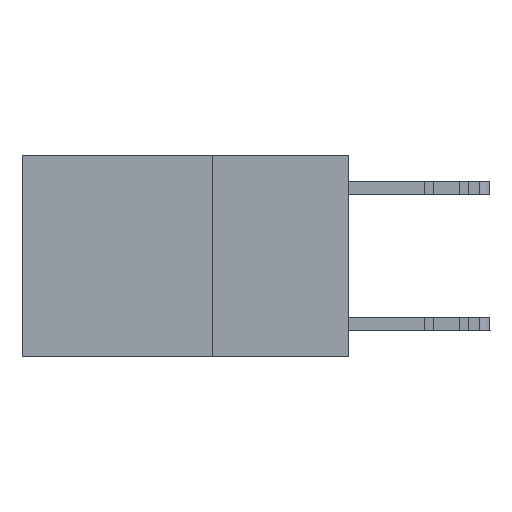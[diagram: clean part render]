
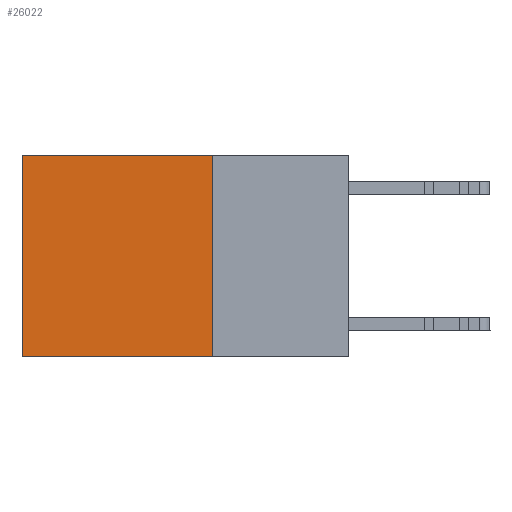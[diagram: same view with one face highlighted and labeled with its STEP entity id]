
A CAD part, left-side view. The second image highlights one B-rep face of the part: STEP entity #26022.
In plain terms, the highlighted planar face has unit normal (-1, 0, 0).
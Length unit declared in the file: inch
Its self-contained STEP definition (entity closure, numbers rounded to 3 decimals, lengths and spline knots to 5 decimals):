
#2023 = CARTESIAN_POINT ( 'NONE',  ( 0.2625, 0.6, 0. ) ) ;
#2108 = PLANE ( 'NONE',  #25555 ) ;
#2206 = ORIENTED_EDGE ( 'NONE', *, *, #14690, .T. ) ;
#4691 = DIRECTION ( 'NONE',  ( 0., 0., -1. ) ) ;
#6877 = ORIENTED_EDGE ( 'NONE', *, *, #31865, .T. ) ;
#6897 = CARTESIAN_POINT ( 'NONE',  ( 0.2625, 0.25, 0. ) ) ;
#7633 = VERTEX_POINT ( 'NONE', #20233 ) ;
#9409 = EDGE_CURVE ( 'NONE', #23916, #25030, #17758, .T. ) ;
#9437 = VERTEX_POINT ( 'NONE', #6897 ) ;
#10968 = LINE ( 'NONE', #23089, #26407 ) ;
#11083 = EDGE_LOOP ( 'NONE', ( #6877, #31672, #31419, #2206 ) ) ;
#12290 = FACE_OUTER_BOUND ( 'NONE', #11083, .T. ) ;
#14148 = DIRECTION ( 'NONE',  ( 0., 0., -1. ) ) ;
#14690 = EDGE_CURVE ( 'NONE', #9437, #7633, #10968, .T. ) ;
#15938 = CARTESIAN_POINT ( 'NONE',  ( 0.2625, 0.25, -0.37 ) ) ;
#16152 = DIRECTION ( 'NONE',  ( 0., 1., 0. ) ) ;
#16973 = VECTOR ( 'NONE', #14148, 39.37008 ) ;
#16997 = CARTESIAN_POINT ( 'NONE',  ( 0.2625, 0.25, 0. ) ) ;
#17758 = LINE ( 'NONE', #23254, #30522 ) ;
#18990 = LINE ( 'NONE', #2023, #16973 ) ;
#20233 = CARTESIAN_POINT ( 'NONE',  ( 0.2625, 0.6, 0. ) ) ;
#22147 = CARTESIAN_POINT ( 'NONE',  ( 0.2625, 0.25, 0. ) ) ;
#23089 = CARTESIAN_POINT ( 'NONE',  ( 0.2625, 0.25, 0. ) ) ;
#23254 = CARTESIAN_POINT ( 'NONE',  ( 0.2625, 0.25, -0.37 ) ) ;
#23916 = VERTEX_POINT ( 'NONE', #15938 ) ;
#25030 = VERTEX_POINT ( 'NONE', #29655 ) ;
#25555 = AXIS2_PLACEMENT_3D ( 'NONE', #22147, #28794, #31704 ) ;
#26022 = ADVANCED_FACE ( 'NONE', ( #12290 ), #2108, .F. ) ;
#26407 = VECTOR ( 'NONE', #16152, 39.37008 ) ;
#27153 = VECTOR ( 'NONE', #4691, 39.37008 ) ;
#27630 = DIRECTION ( 'NONE',  ( 0., 1., 0. ) ) ;
#28622 = EDGE_CURVE ( 'NONE', #9437, #23916, #29434, .T. ) ;
#28794 = DIRECTION ( 'NONE',  ( 1., 0., 0. ) ) ;
#29434 = LINE ( 'NONE', #16997, #27153 ) ;
#29655 = CARTESIAN_POINT ( 'NONE',  ( 0.2625, 0.6, -0.37 ) ) ;
#30522 = VECTOR ( 'NONE', #27630, 39.37008 ) ;
#31419 = ORIENTED_EDGE ( 'NONE', *, *, #28622, .F. ) ;
#31672 = ORIENTED_EDGE ( 'NONE', *, *, #9409, .F. ) ;
#31704 = DIRECTION ( 'NONE',  ( 0., 0., -1. ) ) ;
#31865 = EDGE_CURVE ( 'NONE', #7633, #25030, #18990, .T. ) ;
